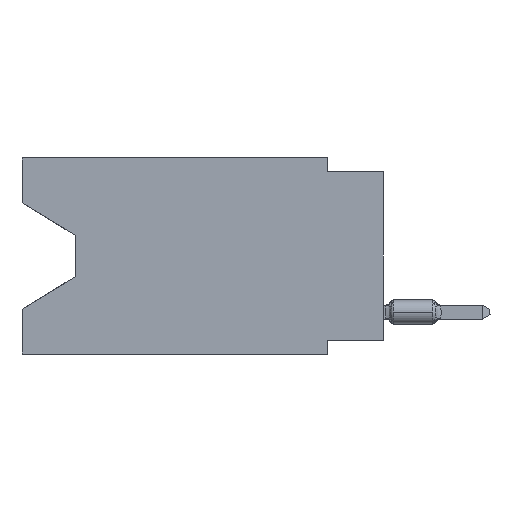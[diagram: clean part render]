
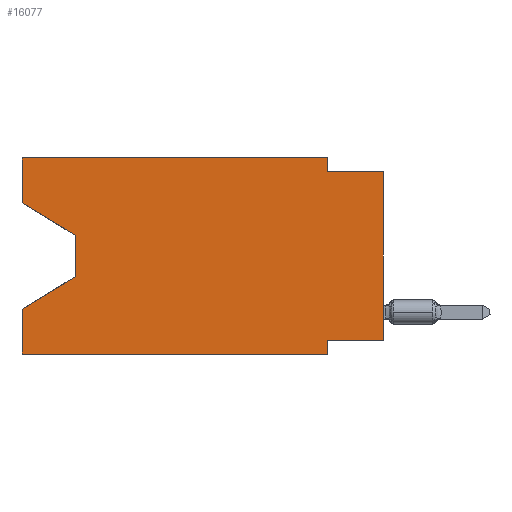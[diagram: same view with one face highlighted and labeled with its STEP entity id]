
A CAD part, left-side view. The second image highlights one B-rep face of the part: STEP entity #16077.
In plain terms, the highlighted planar face has unit normal (-1, 0, 0).
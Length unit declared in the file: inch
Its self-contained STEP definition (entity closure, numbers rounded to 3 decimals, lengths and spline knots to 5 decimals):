
#1635 = VECTOR ( 'NONE', #20386, 39.37008 ) ;
#1766 = EDGE_CURVE ( 'NONE', #19176, #25933, #23766, .T. ) ;
#1915 = DIRECTION ( 'NONE',  ( 0., 0., -1. ) ) ;
#3439 = LINE ( 'NONE', #40933, #31671 ) ;
#4030 = CARTESIAN_POINT ( 'NONE',  ( 0., 0.55, -0.138 ) ) ;
#4300 = VECTOR ( 'NONE', #42716, 39.37008 ) ;
#4603 = VERTEX_POINT ( 'NONE', #23446 ) ;
#4952 = ORIENTED_EDGE ( 'NONE', *, *, #17188, .F. ) ;
#5758 = DIRECTION ( 'NONE',  ( 0., 0., 1. ) ) ;
#6006 = VERTEX_POINT ( 'NONE', #19562 ) ;
#6388 = LINE ( 'NONE', #23916, #41168 ) ;
#6608 = DIRECTION ( 'NONE',  ( 0., 0.855, -0.519 ) ) ;
#6684 = CARTESIAN_POINT ( 'NONE',  ( 0., 0.55, -0.138 ) ) ;
#7607 = VECTOR ( 'NONE', #39330, 39.37008 ) ;
#7985 = ORIENTED_EDGE ( 'NONE', *, *, #33730, .F. ) ;
#8125 = ORIENTED_EDGE ( 'NONE', *, *, #10688, .F. ) ;
#8445 = LINE ( 'NONE', #21914, #12587 ) ;
#8598 = VERTEX_POINT ( 'NONE', #9240 ) ;
#8626 = EDGE_CURVE ( 'NONE', #15532, #8598, #36201, .T. ) ;
#8637 = PLANE ( 'NONE',  #12491 ) ;
#8843 = VECTOR ( 'NONE', #25086, 39.37008 ) ;
#8994 = ORIENTED_EDGE ( 'NONE', *, *, #30065, .F. ) ;
#9240 = CARTESIAN_POINT ( 'NONE',  ( 0., 0.1, -0.35 ) ) ;
#9253 = ORIENTED_EDGE ( 'NONE', *, *, #20104, .F. ) ;
#10166 = DIRECTION ( 'NONE',  ( 0., 0., 1. ) ) ;
#10688 = EDGE_CURVE ( 'NONE', #41552, #26077, #27943, .T. ) ;
#10878 = CARTESIAN_POINT ( 'NONE',  ( 0., 0., -0.025 ) ) ;
#11085 = CARTESIAN_POINT ( 'NONE',  ( 0., 0.55, -0.212 ) ) ;
#11344 = CARTESIAN_POINT ( 'NONE',  ( 0., 0.1, -0.325 ) ) ;
#11471 = LINE ( 'NONE', #42438, #30585 ) ;
#11743 = EDGE_CURVE ( 'NONE', #25933, #36943, #6388, .T. ) ;
#12055 = DIRECTION ( 'NONE',  ( 0., 0., -1. ) ) ;
#12143 = DIRECTION ( 'NONE',  ( 0., -0.855, -0.519 ) ) ;
#12477 = CARTESIAN_POINT ( 'NONE',  ( 0., 0.645, 0. ) ) ;
#12491 = AXIS2_PLACEMENT_3D ( 'NONE', #12477, #22337, #1915 ) ;
#12538 = CARTESIAN_POINT ( 'NONE',  ( 0., 0.645, 0. ) ) ;
#12587 = VECTOR ( 'NONE', #12055, 39.37008 ) ;
#13294 = ORIENTED_EDGE ( 'NONE', *, *, #30941, .F. ) ;
#14189 = VECTOR ( 'NONE', #5758, 39.37008 ) ;
#14866 = ORIENTED_EDGE ( 'NONE', *, *, #43444, .T. ) ;
#15532 = VERTEX_POINT ( 'NONE', #39722 ) ;
#16002 = DIRECTION ( 'NONE',  ( 0., -1., 0. ) ) ;
#16068 = CARTESIAN_POINT ( 'NONE',  ( 0., 0.645, -0.26975 ) ) ;
#16077 = ADVANCED_FACE ( 'NONE', ( #18991 ), #8637, .F. ) ;
#16398 = VERTEX_POINT ( 'NONE', #11344 ) ;
#17033 = LINE ( 'NONE', #23754, #1635 ) ;
#17188 = EDGE_CURVE ( 'NONE', #16398, #8598, #8445, .T. ) ;
#17792 = ORIENTED_EDGE ( 'NONE', *, *, #11743, .T. ) ;
#18210 = CARTESIAN_POINT ( 'NONE',  ( 0., 0.645, -0.08025 ) ) ;
#18991 = FACE_OUTER_BOUND ( 'NONE', #22628, .T. ) ;
#19138 = VERTEX_POINT ( 'NONE', #40864 ) ;
#19176 = VERTEX_POINT ( 'NONE', #4030 ) ;
#19209 = VERTEX_POINT ( 'NONE', #23017 ) ;
#19562 = CARTESIAN_POINT ( 'NONE',  ( 0., 0.1, 0. ) ) ;
#20104 = EDGE_CURVE ( 'NONE', #19138, #19209, #43062, .T. ) ;
#20386 = DIRECTION ( 'NONE',  ( 0., 1., 0. ) ) ;
#20478 = LINE ( 'NONE', #44304, #23193 ) ;
#21914 = CARTESIAN_POINT ( 'NONE',  ( 0., 0.1, -0.35 ) ) ;
#22268 = CARTESIAN_POINT ( 'NONE',  ( 0., 0., -0.025 ) ) ;
#22337 = DIRECTION ( 'NONE',  ( 1., 0., 0. ) ) ;
#22455 = LINE ( 'NONE', #43121, #7607 ) ;
#22628 = EDGE_LOOP ( 'NONE', ( #43515, #33694, #17792, #13294, #37272, #4952, #8994, #14866, #8125, #7985, #39742, #9253 ) ) ;
#23017 = CARTESIAN_POINT ( 'NONE',  ( 0., 0.645, 0. ) ) ;
#23193 = VECTOR ( 'NONE', #16002, 39.37008 ) ;
#23446 = CARTESIAN_POINT ( 'NONE',  ( 0., 0., -0.325 ) ) ;
#23754 = CARTESIAN_POINT ( 'NONE',  ( 0., 0., -0.325 ) ) ;
#23766 = LINE ( 'NONE', #6684, #8843 ) ;
#23916 = CARTESIAN_POINT ( 'NONE',  ( 0., 0.55, -0.212 ) ) ;
#25086 = DIRECTION ( 'NONE',  ( 0., 0., -1. ) ) ;
#25933 = VERTEX_POINT ( 'NONE', #11085 ) ;
#26077 = VERTEX_POINT ( 'NONE', #22268 ) ;
#27536 = VECTOR ( 'NONE', #12143, 39.37008 ) ;
#27792 = CARTESIAN_POINT ( 'NONE',  ( 0., 0.1, -0.025 ) ) ;
#27943 = LINE ( 'NONE', #10878, #43783 ) ;
#30065 = EDGE_CURVE ( 'NONE', #4603, #16398, #17033, .T. ) ;
#30585 = VECTOR ( 'NONE', #36157, 39.37008 ) ;
#30941 = EDGE_CURVE ( 'NONE', #15532, #36943, #3439, .T. ) ;
#31671 = VECTOR ( 'NONE', #10166, 39.37008 ) ;
#32149 = LINE ( 'NONE', #18210, #27536 ) ;
#33694 = ORIENTED_EDGE ( 'NONE', *, *, #1766, .T. ) ;
#33730 = EDGE_CURVE ( 'NONE', #6006, #41552, #11471, .T. ) ;
#34918 = DIRECTION ( 'NONE',  ( 0., -1., 0. ) ) ;
#35714 = EDGE_CURVE ( 'NONE', #19209, #6006, #20478, .T. ) ;
#36157 = DIRECTION ( 'NONE',  ( 0., 0., -1. ) ) ;
#36201 = LINE ( 'NONE', #43146, #4300 ) ;
#36943 = VERTEX_POINT ( 'NONE', #16068 ) ;
#37272 = ORIENTED_EDGE ( 'NONE', *, *, #8626, .T. ) ;
#39330 = DIRECTION ( 'NONE',  ( 0., 0., 1. ) ) ;
#39722 = CARTESIAN_POINT ( 'NONE',  ( 0., 0.645, -0.35 ) ) ;
#39742 = ORIENTED_EDGE ( 'NONE', *, *, #35714, .F. ) ;
#40825 = EDGE_CURVE ( 'NONE', #19138, #19176, #32149, .T. ) ;
#40864 = CARTESIAN_POINT ( 'NONE',  ( 0., 0.645, -0.08025 ) ) ;
#40933 = CARTESIAN_POINT ( 'NONE',  ( 0., 0.645, 0. ) ) ;
#41168 = VECTOR ( 'NONE', #6608, 39.37008 ) ;
#41552 = VERTEX_POINT ( 'NONE', #27792 ) ;
#42438 = CARTESIAN_POINT ( 'NONE',  ( 0., 0.1, 0. ) ) ;
#42716 = DIRECTION ( 'NONE',  ( 0., -1., 0. ) ) ;
#43062 = LINE ( 'NONE', #12538, #14189 ) ;
#43121 = CARTESIAN_POINT ( 'NONE',  ( 0., 0., 0. ) ) ;
#43146 = CARTESIAN_POINT ( 'NONE',  ( 0., 0.645, -0.35 ) ) ;
#43444 = EDGE_CURVE ( 'NONE', #4603, #26077, #22455, .T. ) ;
#43515 = ORIENTED_EDGE ( 'NONE', *, *, #40825, .T. ) ;
#43783 = VECTOR ( 'NONE', #34918, 39.37008 ) ;
#44304 = CARTESIAN_POINT ( 'NONE',  ( 0., 0.645, 0. ) ) ;
